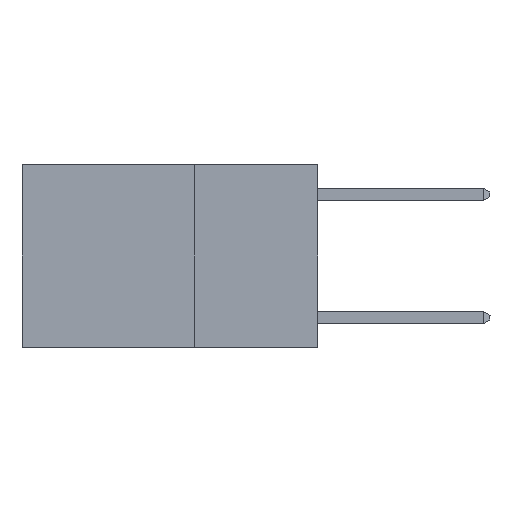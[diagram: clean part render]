
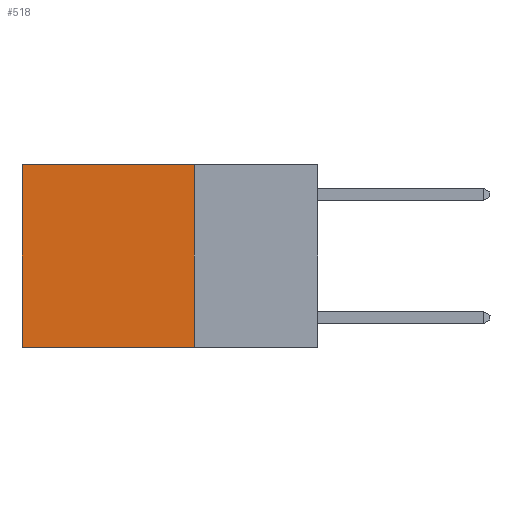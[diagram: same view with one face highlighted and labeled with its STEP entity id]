
A CAD part, left-side view. The second image highlights one B-rep face of the part: STEP entity #518.
In plain terms, the highlighted planar face has unit normal (-1, 0, 0).
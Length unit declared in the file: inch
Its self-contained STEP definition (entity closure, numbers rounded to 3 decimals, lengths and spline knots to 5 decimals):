
#50 = VECTOR ( 'NONE', #10021, 39.37008 ) ;
#425 = CARTESIAN_POINT ( 'NONE',  ( 0.2625, 0.25, 0. ) ) ;
#518 = ADVANCED_FACE ( 'NONE', ( #4421 ), #6109, .F. ) ;
#972 = CARTESIAN_POINT ( 'NONE',  ( 0.2625, 0.6, -0.37 ) ) ;
#1237 = VECTOR ( 'NONE', #1674, 39.37008 ) ;
#1605 = ORIENTED_EDGE ( 'NONE', *, *, #2122, .T. ) ;
#1674 = DIRECTION ( 'NONE',  ( 0., 0., -1. ) ) ;
#1852 = EDGE_LOOP ( 'NONE', ( #1605, #5453, #9355, #6046 ) ) ;
#1863 = VERTEX_POINT ( 'NONE', #425 ) ;
#2122 = EDGE_CURVE ( 'NONE', #4272, #12180, #3096, .T. ) ;
#3096 = LINE ( 'NONE', #8225, #12965 ) ;
#3878 = VECTOR ( 'NONE', #10251, 39.37008 ) ;
#4272 = VERTEX_POINT ( 'NONE', #10043 ) ;
#4421 = FACE_OUTER_BOUND ( 'NONE', #1852, .T. ) ;
#5302 = DIRECTION ( 'NONE',  ( 0., 0., -1. ) ) ;
#5317 = CARTESIAN_POINT ( 'NONE',  ( 0.2625, 0.25, 0. ) ) ;
#5453 = ORIENTED_EDGE ( 'NONE', *, *, #6121, .F. ) ;
#6046 = ORIENTED_EDGE ( 'NONE', *, *, #12975, .T. ) ;
#6109 = PLANE ( 'NONE',  #10868 ) ;
#6121 = EDGE_CURVE ( 'NONE', #12199, #12180, #9938, .T. ) ;
#6246 = LINE ( 'NONE', #7694, #50 ) ;
#6413 = DIRECTION ( 'NONE',  ( 1., 0., 0. ) ) ;
#6781 = LINE ( 'NONE', #10978, #1237 ) ;
#7027 = CARTESIAN_POINT ( 'NONE',  ( 0.2625, 0.25, -0.37 ) ) ;
#7694 = CARTESIAN_POINT ( 'NONE',  ( 0.2625, 0.25, 0. ) ) ;
#8225 = CARTESIAN_POINT ( 'NONE',  ( 0.2625, 0.6, 0. ) ) ;
#8582 = EDGE_CURVE ( 'NONE', #1863, #12199, #6781, .T. ) ;
#9203 = CARTESIAN_POINT ( 'NONE',  ( 0.2625, 0.25, -0.37 ) ) ;
#9355 = ORIENTED_EDGE ( 'NONE', *, *, #8582, .F. ) ;
#9938 = LINE ( 'NONE', #9203, #3878 ) ;
#10021 = DIRECTION ( 'NONE',  ( 0., 1., 0. ) ) ;
#10043 = CARTESIAN_POINT ( 'NONE',  ( 0.2625, 0.6, 0. ) ) ;
#10251 = DIRECTION ( 'NONE',  ( 0., 1., 0. ) ) ;
#10868 = AXIS2_PLACEMENT_3D ( 'NONE', #5317, #6413, #12643 ) ;
#10978 = CARTESIAN_POINT ( 'NONE',  ( 0.2625, 0.25, 0. ) ) ;
#12180 = VERTEX_POINT ( 'NONE', #972 ) ;
#12199 = VERTEX_POINT ( 'NONE', #7027 ) ;
#12643 = DIRECTION ( 'NONE',  ( 0., 0., -1. ) ) ;
#12965 = VECTOR ( 'NONE', #5302, 39.37008 ) ;
#12975 = EDGE_CURVE ( 'NONE', #1863, #4272, #6246, .T. ) ;
